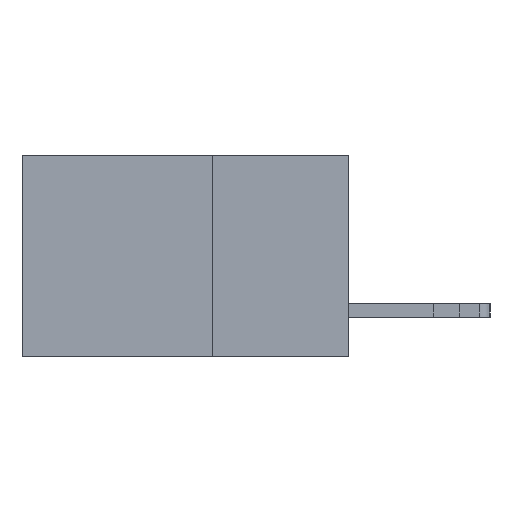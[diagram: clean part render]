
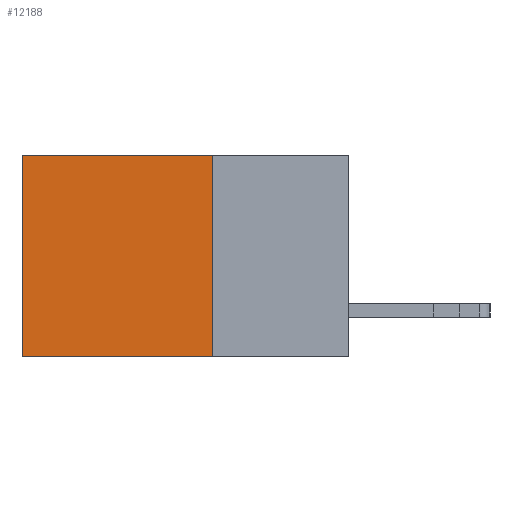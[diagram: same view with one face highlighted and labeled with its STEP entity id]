
A CAD part, left-side view. The second image highlights one B-rep face of the part: STEP entity #12188.
In plain terms, the highlighted planar face has unit normal (-1, 0, 0).
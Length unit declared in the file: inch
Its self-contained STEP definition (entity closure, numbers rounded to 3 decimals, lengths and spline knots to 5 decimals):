
#439 = CARTESIAN_POINT ( 'NONE',  ( 0.298, 0.6, 0. ) ) ;
#465 = DIRECTION ( 'NONE',  ( 0., 0., -1. ) ) ;
#745 = DIRECTION ( 'NONE',  ( 0., 0., -1. ) ) ;
#1039 = LINE ( 'NONE', #21063, #6063 ) ;
#2152 = VERTEX_POINT ( 'NONE', #439 ) ;
#2978 = LINE ( 'NONE', #16959, #6922 ) ;
#3148 = ORIENTED_EDGE ( 'NONE', *, *, #7180, .T. ) ;
#3578 = CARTESIAN_POINT ( 'NONE',  ( 0.298, 0.25, 0. ) ) ;
#4751 = ORIENTED_EDGE ( 'NONE', *, *, #10112, .F. ) ;
#6063 = VECTOR ( 'NONE', #745, 39.37008 ) ;
#6587 = VERTEX_POINT ( 'NONE', #12713 ) ;
#6922 = VECTOR ( 'NONE', #16889, 39.37008 ) ;
#7180 = EDGE_CURVE ( 'NONE', #2152, #11919, #2978, .T. ) ;
#7410 = EDGE_CURVE ( 'NONE', #6587, #2152, #7695, .T. ) ;
#7695 = LINE ( 'NONE', #3578, #15750 ) ;
#8232 = DIRECTION ( 'NONE',  ( 0., 1., 0. ) ) ;
#8907 = CARTESIAN_POINT ( 'NONE',  ( 0.298, 0.25, 0. ) ) ;
#10112 = EDGE_CURVE ( 'NONE', #18512, #11919, #18995, .T. ) ;
#10605 = DIRECTION ( 'NONE',  ( 1., 0., 0. ) ) ;
#11174 = FACE_OUTER_BOUND ( 'NONE', #19338, .T. ) ;
#11607 = CARTESIAN_POINT ( 'NONE',  ( 0.298, 0.25, -0.37 ) ) ;
#11919 = VERTEX_POINT ( 'NONE', #18249 ) ;
#12188 = ADVANCED_FACE ( 'NONE', ( #11174 ), #19117, .F. ) ;
#12267 = ORIENTED_EDGE ( 'NONE', *, *, #7410, .T. ) ;
#12713 = CARTESIAN_POINT ( 'NONE',  ( 0.298, 0.25, 0. ) ) ;
#13573 = EDGE_CURVE ( 'NONE', #6587, #18512, #1039, .T. ) ;
#13960 = VECTOR ( 'NONE', #16130, 39.37008 ) ;
#14382 = CARTESIAN_POINT ( 'NONE',  ( 0.298, 0.25, -0.37 ) ) ;
#15750 = VECTOR ( 'NONE', #8232, 39.37008 ) ;
#16130 = DIRECTION ( 'NONE',  ( 0., 1., 0. ) ) ;
#16889 = DIRECTION ( 'NONE',  ( 0., 0., -1. ) ) ;
#16959 = CARTESIAN_POINT ( 'NONE',  ( 0.298, 0.6, 0. ) ) ;
#18249 = CARTESIAN_POINT ( 'NONE',  ( 0.298, 0.6, -0.37 ) ) ;
#18512 = VERTEX_POINT ( 'NONE', #11607 ) ;
#18995 = LINE ( 'NONE', #14382, #13960 ) ;
#19117 = PLANE ( 'NONE',  #20558 ) ;
#19338 = EDGE_LOOP ( 'NONE', ( #3148, #4751, #20624, #12267 ) ) ;
#20558 = AXIS2_PLACEMENT_3D ( 'NONE', #8907, #10605, #465 ) ;
#20624 = ORIENTED_EDGE ( 'NONE', *, *, #13573, .F. ) ;
#21063 = CARTESIAN_POINT ( 'NONE',  ( 0.298, 0.25, 0. ) ) ;
